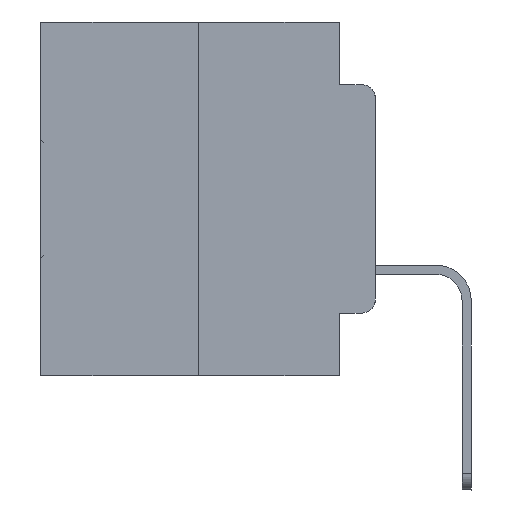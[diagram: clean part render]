
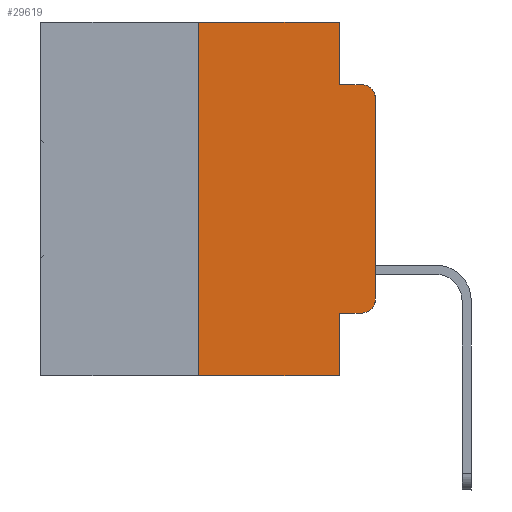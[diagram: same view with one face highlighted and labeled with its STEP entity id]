
A CAD part, left-side view. The second image highlights one B-rep face of the part: STEP entity #29619.
In plain terms, the highlighted planar face has unit normal (-1, 0, 0).
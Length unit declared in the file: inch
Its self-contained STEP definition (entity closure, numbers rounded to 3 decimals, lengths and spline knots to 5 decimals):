
#746 = VECTOR ( 'NONE', #11669, 39.37008 ) ;
#797 = DIRECTION ( 'NONE',  ( 1., 0., 0. ) ) ;
#980 = DIRECTION ( 'NONE',  ( 0., 0., -1. ) ) ;
#1079 = DIRECTION ( 'NONE',  ( -1., 0., 0. ) ) ;
#1285 = DIRECTION ( 'NONE',  ( 0., -1., 0. ) ) ;
#1301 = EDGE_CURVE ( 'NONE', #9358, #5878, #3816, .T. ) ;
#1511 = DIRECTION ( 'NONE',  ( 0., 0., 1. ) ) ;
#2319 = DIRECTION ( 'NONE',  ( 0., 0., -1. ) ) ;
#2393 = VECTOR ( 'NONE', #8216, 39.37008 ) ;
#2868 = CARTESIAN_POINT ( 'NONE',  ( 0., 0.051, -0.4115 ) ) ;
#2881 = VECTOR ( 'NONE', #17743, 39.37008 ) ;
#3755 = VECTOR ( 'NONE', #1285, 39.37008 ) ;
#3816 = LINE ( 'NONE', #23616, #746 ) ;
#3840 = CARTESIAN_POINT ( 'NONE',  ( 0., 0.473, -0.5 ) ) ;
#4350 = CARTESIAN_POINT ( 'NONE',  ( 0., 0.051, 0. ) ) ;
#4351 = EDGE_CURVE ( 'NONE', #31240, #27243, #4418, .T. ) ;
#4418 = LINE ( 'NONE', #7901, #2881 ) ;
#4534 = VECTOR ( 'NONE', #17742, 39.37008 ) ;
#4676 = CARTESIAN_POINT ( 'NONE',  ( 0., 0.051, 0. ) ) ;
#5551 = ORIENTED_EDGE ( 'NONE', *, *, #16962, .T. ) ;
#5878 = VERTEX_POINT ( 'NONE', #28277 ) ;
#6235 = CARTESIAN_POINT ( 'NONE',  ( 0., 0.25, 0. ) ) ;
#6388 = CARTESIAN_POINT ( 'NONE',  ( 0., 0.25, 0. ) ) ;
#6433 = VERTEX_POINT ( 'NONE', #6388 ) ;
#6567 = VERTEX_POINT ( 'NONE', #4350 ) ;
#6727 = ORIENTED_EDGE ( 'NONE', *, *, #8075, .F. ) ;
#7218 = LINE ( 'NONE', #30335, #3755 ) ;
#7515 = LINE ( 'NONE', #6235, #23394 ) ;
#7901 = CARTESIAN_POINT ( 'NONE',  ( 0., 0., 0. ) ) ;
#8075 = EDGE_CURVE ( 'NONE', #9190, #30900, #9674, .T. ) ;
#8113 = CARTESIAN_POINT ( 'NONE',  ( 0., 0.051, -0.0885 ) ) ;
#8216 = DIRECTION ( 'NONE',  ( 0., -1., 0. ) ) ;
#9190 = VERTEX_POINT ( 'NONE', #16130 ) ;
#9358 = VERTEX_POINT ( 'NONE', #14514 ) ;
#9674 = LINE ( 'NONE', #8113, #2393 ) ;
#9937 = ORIENTED_EDGE ( 'NONE', *, *, #14181, .F. ) ;
#10308 = DIRECTION ( 'NONE',  ( 0., 0., -1. ) ) ;
#10383 = AXIS2_PLACEMENT_3D ( 'NONE', #17719, #797, #10308 ) ;
#10441 = ORIENTED_EDGE ( 'NONE', *, *, #4351, .T. ) ;
#10556 = EDGE_CURVE ( 'NONE', #6433, #6567, #7218, .T. ) ;
#11669 = DIRECTION ( 'NONE',  ( 0., 0., -1. ) ) ;
#11801 = CIRCLE ( 'NONE', #13510, 0.02 ) ;
#12005 = CARTESIAN_POINT ( 'NONE',  ( 0., 0.02, -0.4115 ) ) ;
#12476 = VERTEX_POINT ( 'NONE', #12005 ) ;
#12596 = EDGE_CURVE ( 'NONE', #12476, #31240, #25778, .T. ) ;
#12897 = ORIENTED_EDGE ( 'NONE', *, *, #12596, .T. ) ;
#13391 = LINE ( 'NONE', #3840, #21363 ) ;
#13510 = AXIS2_PLACEMENT_3D ( 'NONE', #22944, #1079, #980 ) ;
#13596 = LINE ( 'NONE', #4676, #15918 ) ;
#14181 = EDGE_CURVE ( 'NONE', #25567, #6433, #7515, .T. ) ;
#14514 = CARTESIAN_POINT ( 'NONE',  ( 0., 0.051, -0.4115 ) ) ;
#14759 = CARTESIAN_POINT ( 'NONE',  ( 0., 0.02, -0.3915 ) ) ;
#15469 = CARTESIAN_POINT ( 'NONE',  ( 0., 0.25, -0.5 ) ) ;
#15918 = VECTOR ( 'NONE', #23926, 39.37008 ) ;
#16130 = CARTESIAN_POINT ( 'NONE',  ( 0., 0.051, -0.0885 ) ) ;
#16179 = DIRECTION ( 'NONE',  ( 0., -1., 0. ) ) ;
#16587 = ORIENTED_EDGE ( 'NONE', *, *, #26476, .T. ) ;
#16962 = EDGE_CURVE ( 'NONE', #27243, #30900, #11801, .T. ) ;
#17719 = CARTESIAN_POINT ( 'NONE',  ( 0., 0.473, 0. ) ) ;
#17742 = DIRECTION ( 'NONE',  ( 0., -1., 0. ) ) ;
#17743 = DIRECTION ( 'NONE',  ( 0., 0., 1. ) ) ;
#18006 = EDGE_CURVE ( 'NONE', #9358, #12476, #23845, .T. ) ;
#18312 = CARTESIAN_POINT ( 'NONE',  ( 0., 0.02, -0.0885 ) ) ;
#19440 = DIRECTION ( 'NONE',  ( -1., 0., 0. ) ) ;
#19847 = PLANE ( 'NONE',  #10383 ) ;
#20758 = AXIS2_PLACEMENT_3D ( 'NONE', #14759, #19440, #2319 ) ;
#20834 = EDGE_LOOP ( 'NONE', ( #10441, #5551, #6727, #25054, #23116, #9937, #16587, #31291, #21673, #12897 ) ) ;
#21363 = VECTOR ( 'NONE', #16179, 39.37008 ) ;
#21673 = ORIENTED_EDGE ( 'NONE', *, *, #18006, .T. ) ;
#22944 = CARTESIAN_POINT ( 'NONE',  ( 0., 0.02, -0.1085 ) ) ;
#23116 = ORIENTED_EDGE ( 'NONE', *, *, #10556, .F. ) ;
#23394 = VECTOR ( 'NONE', #1511, 39.37008 ) ;
#23616 = CARTESIAN_POINT ( 'NONE',  ( 0., 0.051, 0. ) ) ;
#23652 = EDGE_CURVE ( 'NONE', #6567, #9190, #13596, .T. ) ;
#23845 = LINE ( 'NONE', #2868, #4534 ) ;
#23926 = DIRECTION ( 'NONE',  ( 0., 0., -1. ) ) ;
#25054 = ORIENTED_EDGE ( 'NONE', *, *, #23652, .F. ) ;
#25567 = VERTEX_POINT ( 'NONE', #15469 ) ;
#25778 = CIRCLE ( 'NONE', #20758, 0.02 ) ;
#26476 = EDGE_CURVE ( 'NONE', #25567, #5878, #13391, .T. ) ;
#26823 = CARTESIAN_POINT ( 'NONE',  ( 0., 0., -0.3915 ) ) ;
#27243 = VERTEX_POINT ( 'NONE', #28999 ) ;
#28277 = CARTESIAN_POINT ( 'NONE',  ( 0., 0.051, -0.5 ) ) ;
#28999 = CARTESIAN_POINT ( 'NONE',  ( 0., 0., -0.1085 ) ) ;
#29617 = FACE_OUTER_BOUND ( 'NONE', #20834, .T. ) ;
#29619 = ADVANCED_FACE ( 'NONE', ( #29617 ), #19847, .F. ) ;
#30335 = CARTESIAN_POINT ( 'NONE',  ( 0., 0.473, 0. ) ) ;
#30900 = VERTEX_POINT ( 'NONE', #18312 ) ;
#31240 = VERTEX_POINT ( 'NONE', #26823 ) ;
#31291 = ORIENTED_EDGE ( 'NONE', *, *, #1301, .F. ) ;
